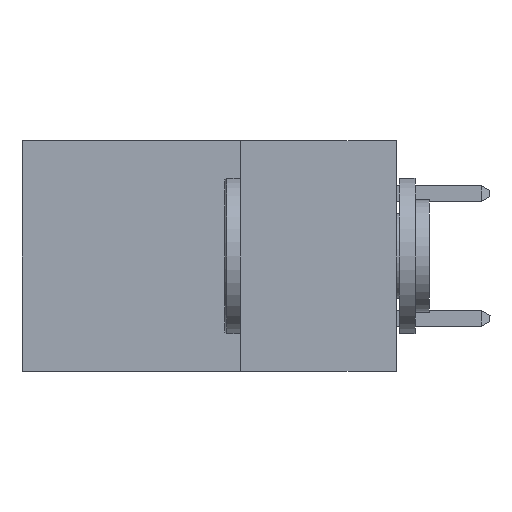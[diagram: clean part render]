
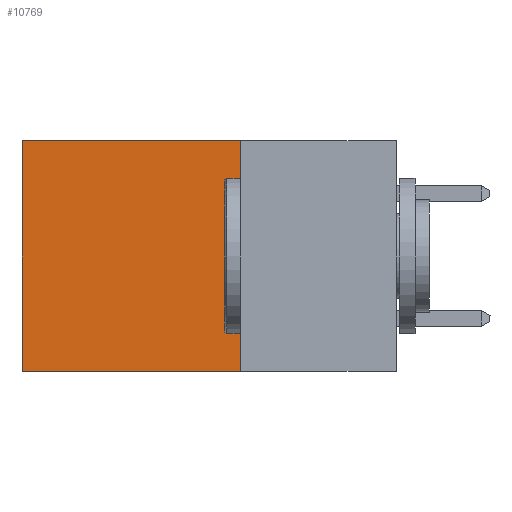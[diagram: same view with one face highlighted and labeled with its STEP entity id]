
A CAD part, left-side view. The second image highlights one B-rep face of the part: STEP entity #10769.
In plain terms, the highlighted planar face has unit normal (-1, 0, 0).
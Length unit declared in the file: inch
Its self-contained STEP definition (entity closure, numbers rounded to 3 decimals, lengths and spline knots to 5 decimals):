
#889 = LINE ( 'NONE', #4805, #5888 ) ;
#968 = VERTEX_POINT ( 'NONE', #2844 ) ;
#1669 = EDGE_CURVE ( 'NONE', #6780, #968, #889, .T. ) ;
#1684 = VERTEX_POINT ( 'NONE', #8686 ) ;
#1781 = VECTOR ( 'NONE', #13175, 39.37008 ) ;
#2040 = CARTESIAN_POINT ( 'NONE',  ( 0.2615, 0.25, 0. ) ) ;
#2091 = DIRECTION ( 'NONE',  ( 0., 1., 0. ) ) ;
#2390 = CARTESIAN_POINT ( 'NONE',  ( 0.2615, 0.6, -0.37 ) ) ;
#2844 = CARTESIAN_POINT ( 'NONE',  ( 0.2615, 0.6, -0.37 ) ) ;
#3736 = DIRECTION ( 'NONE',  ( 0., 0., -1. ) ) ;
#4447 = EDGE_CURVE ( 'NONE', #11871, #968, #5290, .T. ) ;
#4514 = EDGE_CURVE ( 'NONE', #1684, #6780, #10104, .T. ) ;
#4799 = DIRECTION ( 'NONE',  ( 0., 1., 0. ) ) ;
#4805 = CARTESIAN_POINT ( 'NONE',  ( 0.2615, 0.25, -0.37 ) ) ;
#5290 = LINE ( 'NONE', #2390, #12962 ) ;
#5647 = VECTOR ( 'NONE', #2091, 39.37008 ) ;
#5888 = VECTOR ( 'NONE', #4799, 39.37008 ) ;
#6730 = CARTESIAN_POINT ( 'NONE',  ( 0.2615, 0.6, 0. ) ) ;
#6780 = VERTEX_POINT ( 'NONE', #7068 ) ;
#7068 = CARTESIAN_POINT ( 'NONE',  ( 0.2615, 0.25, -0.37 ) ) ;
#7739 = ORIENTED_EDGE ( 'NONE', *, *, #4447, .T. ) ;
#7749 = ORIENTED_EDGE ( 'NONE', *, *, #1669, .F. ) ;
#7761 = ORIENTED_EDGE ( 'NONE', *, *, #4514, .F. ) ;
#7827 = ORIENTED_EDGE ( 'NONE', *, *, #12166, .T. ) ;
#8282 = DIRECTION ( 'NONE',  ( 0., 0., -1. ) ) ;
#8296 = DIRECTION ( 'NONE',  ( 1., 0., 0. ) ) ;
#8435 = PLANE ( 'NONE',  #10288 ) ;
#8460 = CARTESIAN_POINT ( 'NONE',  ( 0.2615, 0.25, -0.37 ) ) ;
#8686 = CARTESIAN_POINT ( 'NONE',  ( 0.2615, 0.25, 0. ) ) ;
#9055 = EDGE_LOOP ( 'NONE', ( #7739, #7749, #7761, #7827 ) ) ;
#10104 = LINE ( 'NONE', #13270, #1781 ) ;
#10288 = AXIS2_PLACEMENT_3D ( 'NONE', #8460, #8296, #8282 ) ;
#10769 = ADVANCED_FACE ( 'NONE', ( #11242 ), #8435, .F. ) ;
#11068 = LINE ( 'NONE', #2040, #5647 ) ;
#11242 = FACE_OUTER_BOUND ( 'NONE', #9055, .T. ) ;
#11871 = VERTEX_POINT ( 'NONE', #6730 ) ;
#12166 = EDGE_CURVE ( 'NONE', #1684, #11871, #11068, .T. ) ;
#12962 = VECTOR ( 'NONE', #3736, 39.37008 ) ;
#13175 = DIRECTION ( 'NONE',  ( 0., 0., -1. ) ) ;
#13270 = CARTESIAN_POINT ( 'NONE',  ( 0.2615, 0.25, -0.37 ) ) ;
